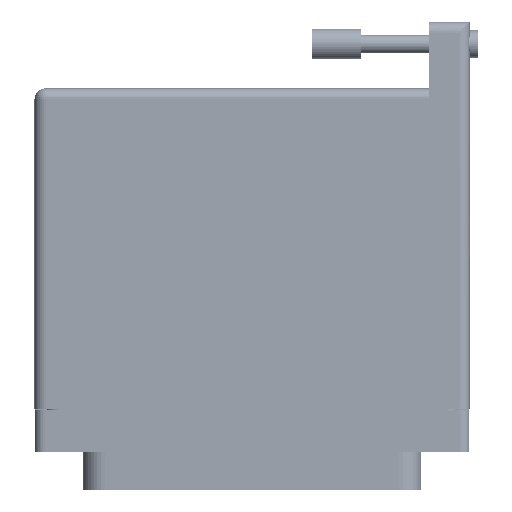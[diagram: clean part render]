
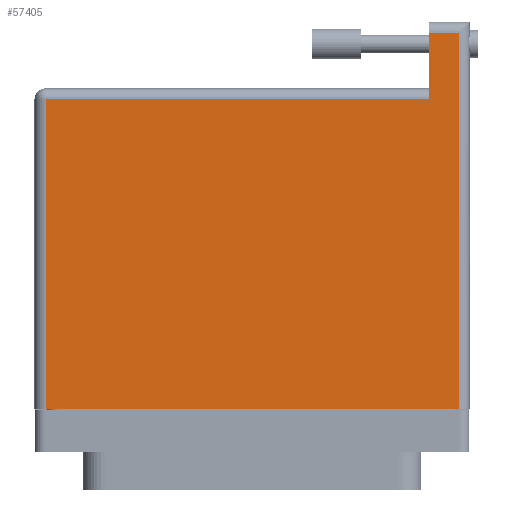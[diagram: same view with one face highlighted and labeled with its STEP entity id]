
A CAD part, front view. The second image highlights one B-rep face of the part: STEP entity #57405.
In plain terms, the highlighted face is planar.
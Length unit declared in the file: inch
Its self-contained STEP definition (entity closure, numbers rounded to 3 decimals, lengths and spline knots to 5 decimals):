
#60 = VECTOR ( 'NONE', #3306, 39.37008 ) ;
#898 = ORIENTED_EDGE ( 'NONE', *, *, #91680, .T. ) ;
#3306 = DIRECTION ( 'NONE',  ( 0., -1., 0. ) ) ;
#3566 = CARTESIAN_POINT ( 'NONE',  ( 1.3075, 2.35, 0.765 ) ) ;
#3584 = EDGE_LOOP ( 'NONE', ( #72565, #8614, #9855, #30553, #898, #82082 ) ) ;
#3947 = FACE_OUTER_BOUND ( 'NONE', #3584, .T. ) ;
#4276 = EDGE_CURVE ( 'NONE', #84343, #20878, #91809, .T. ) ;
#5602 = LINE ( 'NONE', #73370, #23376 ) ;
#6000 = VERTEX_POINT ( 'NONE', #67107 ) ;
#7504 = VECTOR ( 'NONE', #36936, 39.37008 ) ;
#8614 = ORIENTED_EDGE ( 'NONE', *, *, #29652, .T. ) ;
#9409 = EDGE_CURVE ( 'NONE', #6000, #39505, #5602, .T. ) ;
#9855 = ORIENTED_EDGE ( 'NONE', *, *, #9409, .T. ) ;
#11086 = DIRECTION ( 'NONE',  ( -1., 0., 0. ) ) ;
#18846 = CARTESIAN_POINT ( 'NONE',  ( -1.3775, 1.93, 0.765 ) ) ;
#20878 = VERTEX_POINT ( 'NONE', #92074 ) ;
#23376 = VECTOR ( 'NONE', #81517, 39.37008 ) ;
#24248 = CARTESIAN_POINT ( 'NONE',  ( 1.1215, 2.35, 0.765 ) ) ;
#24558 = DIRECTION ( 'NONE',  ( -1., 0., 0. ) ) ;
#25192 = CARTESIAN_POINT ( 'NONE',  ( -1.3775, 1.86, 0.765 ) ) ;
#29652 = EDGE_CURVE ( 'NONE', #20878, #6000, #42617, .T. ) ;
#30553 = ORIENTED_EDGE ( 'NONE', *, *, #91956, .T. ) ;
#31378 = VECTOR ( 'NONE', #11086, 39.37008 ) ;
#32947 = PLANE ( 'NONE',  #85837 ) ;
#36936 = DIRECTION ( 'NONE',  ( 1., 0., 0. ) ) ;
#37677 = VERTEX_POINT ( 'NONE', #56108 ) ;
#39505 = VERTEX_POINT ( 'NONE', #69383 ) ;
#40811 = DIRECTION ( 'NONE',  ( -1., 0., 0. ) ) ;
#42617 = LINE ( 'NONE', #25192, #31378 ) ;
#44854 = CARTESIAN_POINT ( 'NONE',  ( 1.3075, 2.28, 0.765 ) ) ;
#53103 = LINE ( 'NONE', #73088, #58751 ) ;
#56108 = CARTESIAN_POINT ( 'NONE',  ( 1.3075, -0.1, 0.765 ) ) ;
#57405 = ADVANCED_FACE ( 'NONE', ( #3947 ), #32947, .F. ) ;
#58751 = VECTOR ( 'NONE', #24558, 39.37008 ) ;
#63114 = EDGE_CURVE ( 'NONE', #91020, #84343, #53103, .T. ) ;
#67107 = CARTESIAN_POINT ( 'NONE',  ( -1.3075, 1.86, 0.765 ) ) ;
#67391 = DIRECTION ( 'NONE',  ( 0., 1., 0. ) ) ;
#68935 = DIRECTION ( 'NONE',  ( 0., 0., -1. ) ) ;
#69383 = CARTESIAN_POINT ( 'NONE',  ( -1.3075, -0.1, 0.765 ) ) ;
#72565 = ORIENTED_EDGE ( 'NONE', *, *, #4276, .T. ) ;
#73088 = CARTESIAN_POINT ( 'NONE',  ( -1.3775, 2.28, 0.765 ) ) ;
#73370 = CARTESIAN_POINT ( 'NONE',  ( -1.3075, -0.1, 0.765 ) ) ;
#81517 = DIRECTION ( 'NONE',  ( 0., -1., 0. ) ) ;
#82082 = ORIENTED_EDGE ( 'NONE', *, *, #63114, .T. ) ;
#82574 = VECTOR ( 'NONE', #67391, 39.37008 ) ;
#84343 = VERTEX_POINT ( 'NONE', #85584 ) ;
#85584 = CARTESIAN_POINT ( 'NONE',  ( 1.1215, 2.28, 0.765 ) ) ;
#85837 = AXIS2_PLACEMENT_3D ( 'NONE', #18846, #68935, #40811 ) ;
#87020 = CARTESIAN_POINT ( 'NONE',  ( -1.3775, -0.1, 0.765 ) ) ;
#90327 = LINE ( 'NONE', #87020, #7504 ) ;
#91020 = VERTEX_POINT ( 'NONE', #44854 ) ;
#91505 = LINE ( 'NONE', #3566, #82574 ) ;
#91680 = EDGE_CURVE ( 'NONE', #37677, #91020, #91505, .T. ) ;
#91809 = LINE ( 'NONE', #24248, #60 ) ;
#91956 = EDGE_CURVE ( 'NONE', #39505, #37677, #90327, .T. ) ;
#92074 = CARTESIAN_POINT ( 'NONE',  ( 1.1215, 1.86, 0.765 ) ) ;
